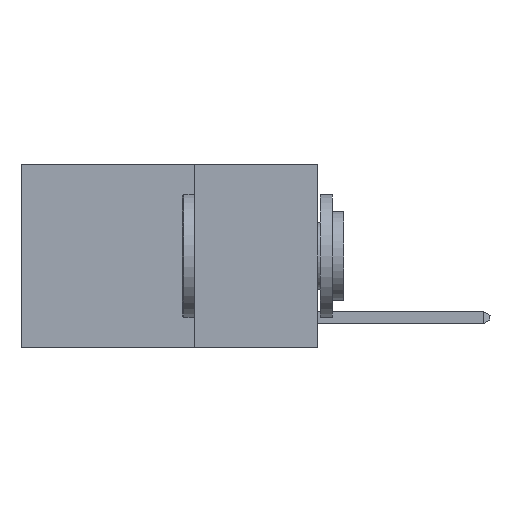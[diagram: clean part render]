
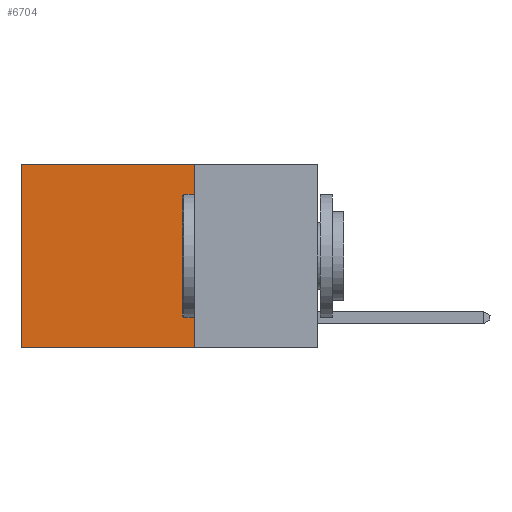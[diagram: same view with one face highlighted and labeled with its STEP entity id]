
A CAD part, left-side view. The second image highlights one B-rep face of the part: STEP entity #6704.
In plain terms, the highlighted planar face has unit normal (-1, 0, 0).
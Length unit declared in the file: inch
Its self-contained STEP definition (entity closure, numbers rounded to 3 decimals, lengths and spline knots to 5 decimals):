
#84 = EDGE_CURVE ( 'NONE', #4310, #25479, #1169, .T. ) ;
#1169 = LINE ( 'NONE', #26196, #10861 ) ;
#2217 = ORIENTED_EDGE ( 'NONE', *, *, #2617, .F. ) ;
#2331 = VECTOR ( 'NONE', #16034, 39.37008 ) ;
#2617 = EDGE_CURVE ( 'NONE', #27087, #4310, #5564, .T. ) ;
#2691 = EDGE_CURVE ( 'NONE', #21629, #25479, #14433, .T. ) ;
#4310 = VERTEX_POINT ( 'NONE', #24394 ) ;
#5030 = VECTOR ( 'NONE', #7191, 39.37008 ) ;
#5564 = LINE ( 'NONE', #21204, #5030 ) ;
#5704 = PLANE ( 'NONE',  #26801 ) ;
#6704 = ADVANCED_FACE ( 'NONE', ( #7909 ), #5704, .F. ) ;
#7191 = DIRECTION ( 'NONE',  ( 0., 0., -1. ) ) ;
#7909 = FACE_OUTER_BOUND ( 'NONE', #19948, .T. ) ;
#10272 = CARTESIAN_POINT ( 'NONE',  ( 0.2625, 0.25, 0. ) ) ;
#10861 = VECTOR ( 'NONE', #12628, 39.37008 ) ;
#12628 = DIRECTION ( 'NONE',  ( 0., 1., 0. ) ) ;
#13061 = EDGE_CURVE ( 'NONE', #27087, #21629, #23245, .T. ) ;
#14433 = LINE ( 'NONE', #24304, #15869 ) ;
#15159 = DIRECTION ( 'NONE',  ( 0., 0., -1. ) ) ;
#15706 = CARTESIAN_POINT ( 'NONE',  ( 0.2625, 0.6, -0.37 ) ) ;
#15869 = VECTOR ( 'NONE', #15159, 39.37008 ) ;
#16034 = DIRECTION ( 'NONE',  ( 0., 1., 0. ) ) ;
#18740 = ORIENTED_EDGE ( 'NONE', *, *, #13061, .T. ) ;
#19948 = EDGE_LOOP ( 'NONE', ( #20558, #22872, #2217, #18740 ) ) ;
#20558 = ORIENTED_EDGE ( 'NONE', *, *, #2691, .T. ) ;
#21204 = CARTESIAN_POINT ( 'NONE',  ( 0.2625, 0.25, 0. ) ) ;
#21629 = VERTEX_POINT ( 'NONE', #26062 ) ;
#22872 = ORIENTED_EDGE ( 'NONE', *, *, #84, .F. ) ;
#23245 = LINE ( 'NONE', #27230, #2331 ) ;
#23407 = DIRECTION ( 'NONE',  ( 1., 0., 0. ) ) ;
#24304 = CARTESIAN_POINT ( 'NONE',  ( 0.2625, 0.6, 0. ) ) ;
#24394 = CARTESIAN_POINT ( 'NONE',  ( 0.2625, 0.25, -0.37 ) ) ;
#25479 = VERTEX_POINT ( 'NONE', #15706 ) ;
#26062 = CARTESIAN_POINT ( 'NONE',  ( 0.2625, 0.6, 0. ) ) ;
#26152 = CARTESIAN_POINT ( 'NONE',  ( 0.2625, 0.25, 0. ) ) ;
#26196 = CARTESIAN_POINT ( 'NONE',  ( 0.2625, 0.25, -0.37 ) ) ;
#26801 = AXIS2_PLACEMENT_3D ( 'NONE', #10272, #23407, #28275 ) ;
#27087 = VERTEX_POINT ( 'NONE', #26152 ) ;
#27230 = CARTESIAN_POINT ( 'NONE',  ( 0.2625, 0.25, 0. ) ) ;
#28275 = DIRECTION ( 'NONE',  ( 0., 0., -1. ) ) ;
